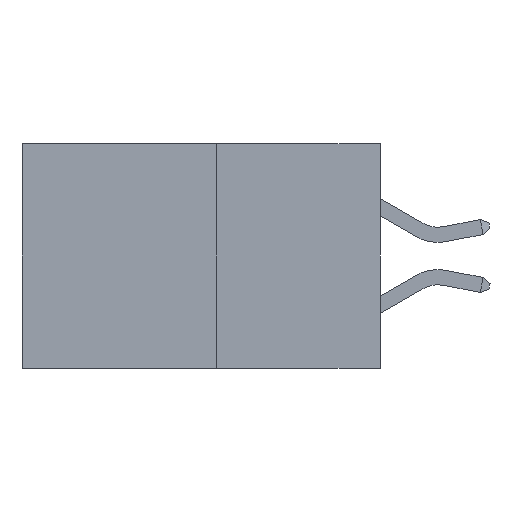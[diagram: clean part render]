
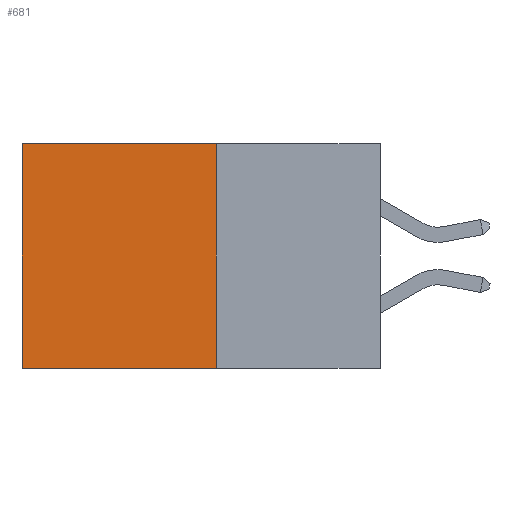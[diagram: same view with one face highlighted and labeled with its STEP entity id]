
A CAD part, left-side view. The second image highlights one B-rep face of the part: STEP entity #681.
In plain terms, the highlighted planar face has unit normal (-1, 0, 0).
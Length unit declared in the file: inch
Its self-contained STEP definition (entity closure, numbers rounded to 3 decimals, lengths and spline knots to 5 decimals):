
#145 = ORIENTED_EDGE ( 'NONE', *, *, #7051, .T. ) ;
#665 = EDGE_CURVE ( 'NONE', #1265, #5022, #10978, .T. ) ;
#681 = ADVANCED_FACE ( 'NONE', ( #4153 ), #10384, .F. ) ;
#1239 = EDGE_CURVE ( 'NONE', #7168, #1265, #2944, .T. ) ;
#1265 = VERTEX_POINT ( 'NONE', #5078 ) ;
#1354 = DIRECTION ( 'NONE',  ( 0., 1., 0. ) ) ;
#1474 = CARTESIAN_POINT ( 'NONE',  ( 0.277, 0.59, -0.37 ) ) ;
#1953 = VERTEX_POINT ( 'NONE', #8389 ) ;
#2573 = CARTESIAN_POINT ( 'NONE',  ( 0.277, 0.27, 0. ) ) ;
#2667 = EDGE_CURVE ( 'NONE', #1953, #5022, #6983, .T. ) ;
#2763 = AXIS2_PLACEMENT_3D ( 'NONE', #7344, #9638, #8035 ) ;
#2886 = EDGE_LOOP ( 'NONE', ( #4108, #8760, #10876, #145 ) ) ;
#2944 = LINE ( 'NONE', #7142, #9586 ) ;
#4108 = ORIENTED_EDGE ( 'NONE', *, *, #2667, .T. ) ;
#4153 = FACE_OUTER_BOUND ( 'NONE', #2886, .T. ) ;
#4831 = VECTOR ( 'NONE', #11050, 39.37008 ) ;
#5022 = VERTEX_POINT ( 'NONE', #1474 ) ;
#5078 = CARTESIAN_POINT ( 'NONE',  ( 0.277, 0.27, -0.37 ) ) ;
#5761 = CARTESIAN_POINT ( 'NONE',  ( 0.277, 0.59, -0.37 ) ) ;
#6087 = LINE ( 'NONE', #6929, #7922 ) ;
#6511 = VECTOR ( 'NONE', #10398, 39.37008 ) ;
#6929 = CARTESIAN_POINT ( 'NONE',  ( 0.277, 0.27, 0. ) ) ;
#6983 = LINE ( 'NONE', #5761, #4831 ) ;
#7051 = EDGE_CURVE ( 'NONE', #7168, #1953, #6087, .T. ) ;
#7142 = CARTESIAN_POINT ( 'NONE',  ( 0.277, 0.27, -0.37 ) ) ;
#7168 = VERTEX_POINT ( 'NONE', #2573 ) ;
#7215 = DIRECTION ( 'NONE',  ( 0., 0., -1. ) ) ;
#7344 = CARTESIAN_POINT ( 'NONE',  ( 0.277, 0.27, -0.37 ) ) ;
#7922 = VECTOR ( 'NONE', #1354, 39.37008 ) ;
#8035 = DIRECTION ( 'NONE',  ( 0., 0., -1. ) ) ;
#8389 = CARTESIAN_POINT ( 'NONE',  ( 0.277, 0.59, 0. ) ) ;
#8760 = ORIENTED_EDGE ( 'NONE', *, *, #665, .F. ) ;
#9586 = VECTOR ( 'NONE', #7215, 39.37008 ) ;
#9638 = DIRECTION ( 'NONE',  ( 1., 0., 0. ) ) ;
#10243 = CARTESIAN_POINT ( 'NONE',  ( 0.277, 0.27, -0.37 ) ) ;
#10384 = PLANE ( 'NONE',  #2763 ) ;
#10398 = DIRECTION ( 'NONE',  ( 0., 1., 0. ) ) ;
#10876 = ORIENTED_EDGE ( 'NONE', *, *, #1239, .F. ) ;
#10978 = LINE ( 'NONE', #10243, #6511 ) ;
#11050 = DIRECTION ( 'NONE',  ( 0., 0., -1. ) ) ;
